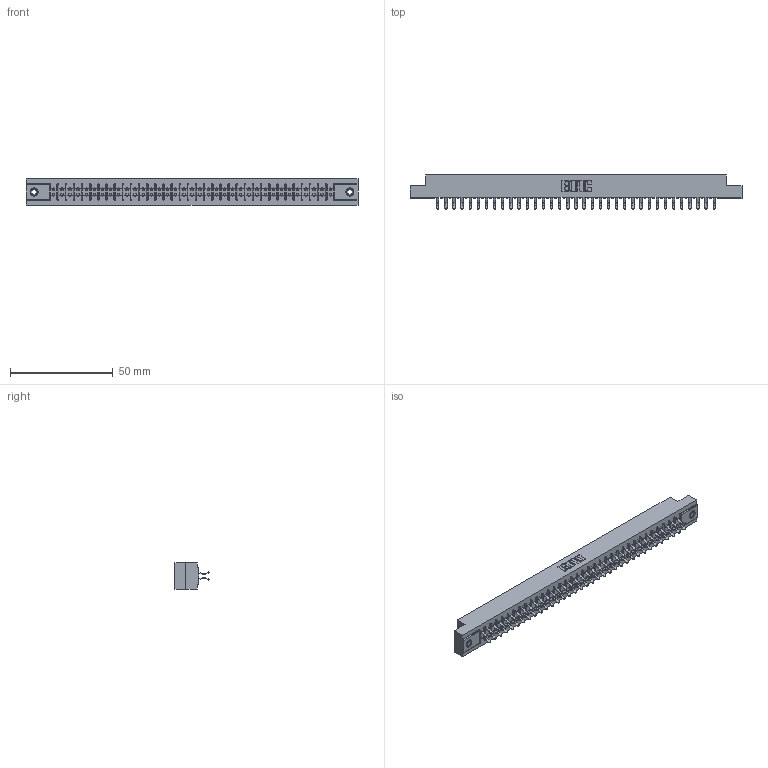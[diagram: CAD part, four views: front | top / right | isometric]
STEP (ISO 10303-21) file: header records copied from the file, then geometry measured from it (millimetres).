
FILE_DESCRIPTION (( 'STEP AP203' ), '1' );
FILE_NAME ('355-070-556-508.STEP', '2019-09-12T17:47:52', ( '' ), ( '' ), 'SwSTEP 2.0', 'SolidWorks 2016', '' );
FILE_SCHEMA (( 'CONFIG_CONTROL_DESIGN' ));
Length unit declared in the file: inch
Products named in the file (4): 305 Part_.156 Dia; 355-070-556-508; 345-250-001_345-250-003-102; 305-290-001_556
Assembly tree (73 placements, depth 2):
  355-070-556-508
    305 Part_.156 Dia
    305-290-001_556  x70
    345-250-001_345-250-003-102  x2
Bounding box: 161.7 x 16.64 x 12.7 mm (x, y, z)
Volume: 16325.4 mm3; surface area: 21429.1 mm2
Topology: 73 solids, 73 shells, 4096 faces, 11757 edges, 7642 vertices
Faces by surface type: plane 2270, cylinder 1670, sphere 140, cone 12, torus 4
Entity records: 40155 total; most frequent: CARTESIAN_POINT 6630, ORIENTED_EDGE 6574, DIRECTION 6433, EDGE_CURVE 3287, LINE 2643, VECTOR 2643, VERTEX_POINT 2092, AXIS2_PLACEMENT_3D 1895
